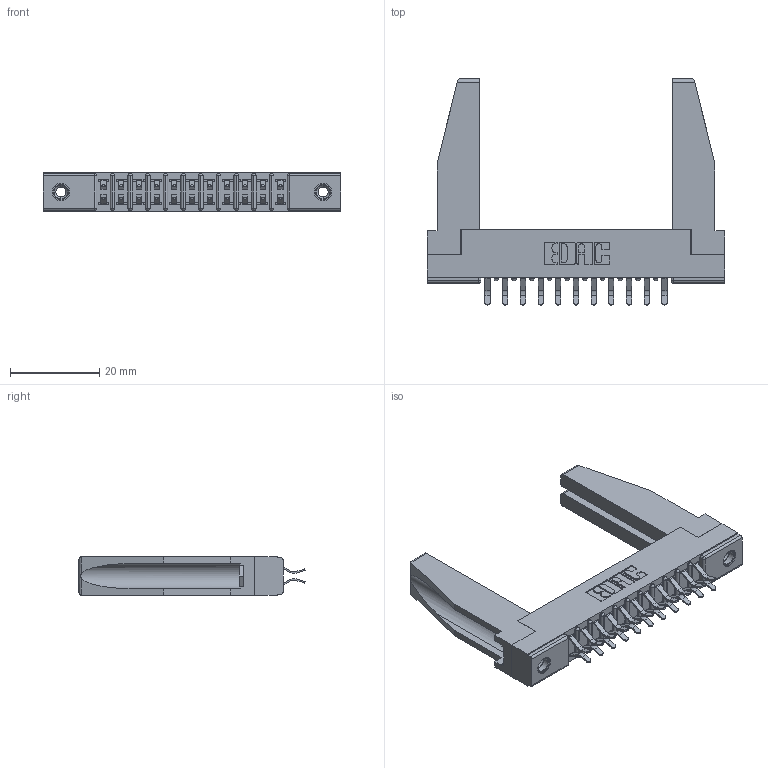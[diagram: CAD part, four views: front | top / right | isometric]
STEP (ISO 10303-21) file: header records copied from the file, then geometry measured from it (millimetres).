
FILE_DESCRIPTION (( 'STEP AP203' ), '1' );
FILE_NAME ('307-022-456-278.STEP', '2020-09-29T04:01:45', ( '' ), ( '' ), 'SwSTEP 2.0', 'SolidWorks 2020', '' );
FILE_SCHEMA (( 'CONFIG_CONTROL_DESIGN' ));
Length unit declared in the file: inch
Products named in the file (5): 345-250-001_345-250-001-102; 307-220-078; 307 Part_.156 Dia Mounting Holes; 307-022-456-278; 307-290-001_556
Assembly tree (27 placements, depth 2):
  307-022-456-278
    307 Part_.156 Dia Mounting Holes
    307-290-001_556  x22
    307-220-078  x2
    345-250-001_345-250-001-102  x2
Bounding box: 66.6 x 50.67 x 8.71 mm (x, y, z)
Volume: 8346.8 mm3; surface area: 10917.8 mm2
Topology: 27 solids, 27 shells, 1360 faces, 3777 edges, 2446 vertices
Faces by surface type: plane 880, cylinder 440, sphere 24, cone 12, torus 4
Entity records: 16147 total; most frequent: CARTESIAN_POINT 2661, ORIENTED_EDGE 2592, DIRECTION 2574, EDGE_CURVE 1296, VECTOR 984, LINE 984, VERTEX_POINT 840, AXIS2_PLACEMENT_3D 795
